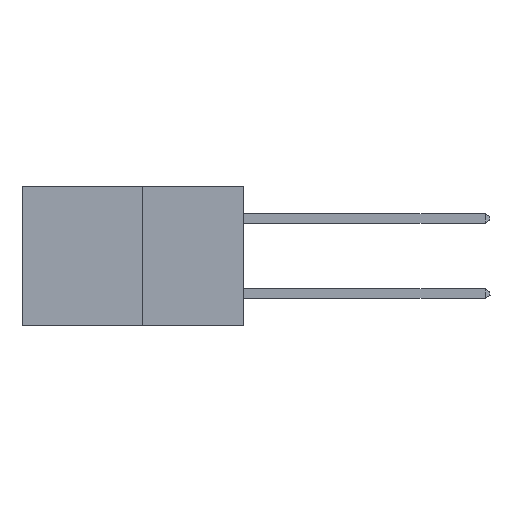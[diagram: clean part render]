
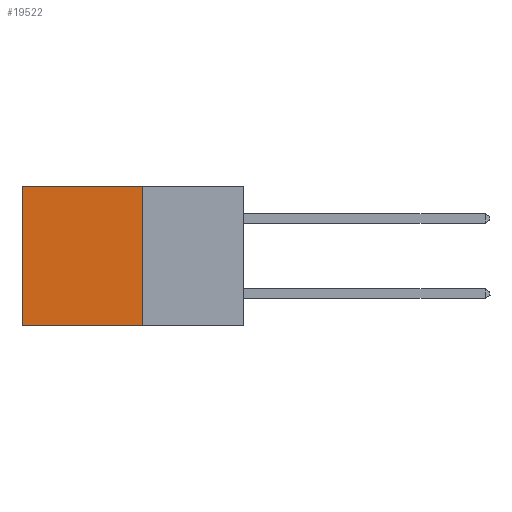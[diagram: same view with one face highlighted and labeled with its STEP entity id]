
A CAD part, left-side view. The second image highlights one B-rep face of the part: STEP entity #19522.
In plain terms, the highlighted planar face has unit normal (-1, 0, 0).
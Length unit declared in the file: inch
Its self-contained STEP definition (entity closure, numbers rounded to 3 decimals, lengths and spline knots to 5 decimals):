
#318 = ORIENTED_EDGE ( 'NONE', *, *, #21920, .T. ) ;
#3483 = LINE ( 'NONE', #23016, #16154 ) ;
#4454 = EDGE_CURVE ( 'NONE', #19556, #29174, #10545, .T. ) ;
#10545 = LINE ( 'NONE', #31183, #23954 ) ;
#11007 = VECTOR ( 'NONE', #30260, 39.37008 ) ;
#11062 = CARTESIAN_POINT ( 'NONE',  ( 0.277, 0.27, -0.37 ) ) ;
#11208 = PLANE ( 'NONE',  #12464 ) ;
#11736 = EDGE_LOOP ( 'NONE', ( #318, #13651, #28528, #15846 ) ) ;
#12286 = VECTOR ( 'NONE', #21292, 39.37008 ) ;
#12464 = AXIS2_PLACEMENT_3D ( 'NONE', #16500, #29898, #13929 ) ;
#12975 = CARTESIAN_POINT ( 'NONE',  ( 0.277, 0.59, 0. ) ) ;
#13651 = ORIENTED_EDGE ( 'NONE', *, *, #26043, .F. ) ;
#13929 = DIRECTION ( 'NONE',  ( 0., 0., -1. ) ) ;
#15846 = ORIENTED_EDGE ( 'NONE', *, *, #31035, .T. ) ;
#16154 = VECTOR ( 'NONE', #28370, 39.37008 ) ;
#16500 = CARTESIAN_POINT ( 'NONE',  ( 0.277, 0.27, -0.37 ) ) ;
#18318 = VERTEX_POINT ( 'NONE', #28003 ) ;
#19401 = LINE ( 'NONE', #23851, #12286 ) ;
#19522 = ADVANCED_FACE ( 'NONE', ( #29510 ), #11208, .F. ) ;
#19556 = VERTEX_POINT ( 'NONE', #27333 ) ;
#21292 = DIRECTION ( 'NONE',  ( 0., 0., -1. ) ) ;
#21920 = EDGE_CURVE ( 'NONE', #31441, #18318, #19401, .T. ) ;
#23016 = CARTESIAN_POINT ( 'NONE',  ( 0.277, 0.27, -0.37 ) ) ;
#23851 = CARTESIAN_POINT ( 'NONE',  ( 0.277, 0.59, -0.37 ) ) ;
#23954 = VECTOR ( 'NONE', #31118, 39.37008 ) ;
#26043 = EDGE_CURVE ( 'NONE', #29174, #18318, #3483, .T. ) ;
#27333 = CARTESIAN_POINT ( 'NONE',  ( 0.277, 0.27, 0. ) ) ;
#27578 = CARTESIAN_POINT ( 'NONE',  ( 0.277, 0.27, 0. ) ) ;
#28003 = CARTESIAN_POINT ( 'NONE',  ( 0.277, 0.59, -0.37 ) ) ;
#28370 = DIRECTION ( 'NONE',  ( 0., 1., 0. ) ) ;
#28528 = ORIENTED_EDGE ( 'NONE', *, *, #4454, .F. ) ;
#29174 = VERTEX_POINT ( 'NONE', #11062 ) ;
#29510 = FACE_OUTER_BOUND ( 'NONE', #11736, .T. ) ;
#29898 = DIRECTION ( 'NONE',  ( 1., 0., 0. ) ) ;
#30260 = DIRECTION ( 'NONE',  ( 0., 1., 0. ) ) ;
#31035 = EDGE_CURVE ( 'NONE', #19556, #31441, #32261, .T. ) ;
#31118 = DIRECTION ( 'NONE',  ( 0., 0., -1. ) ) ;
#31183 = CARTESIAN_POINT ( 'NONE',  ( 0.277, 0.27, -0.37 ) ) ;
#31441 = VERTEX_POINT ( 'NONE', #12975 ) ;
#32261 = LINE ( 'NONE', #27578, #11007 ) ;
